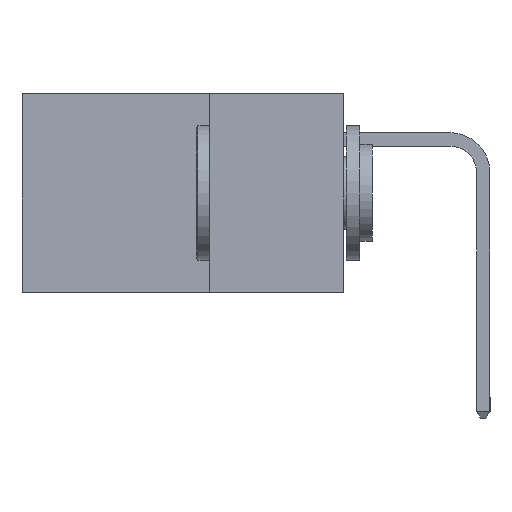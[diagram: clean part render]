
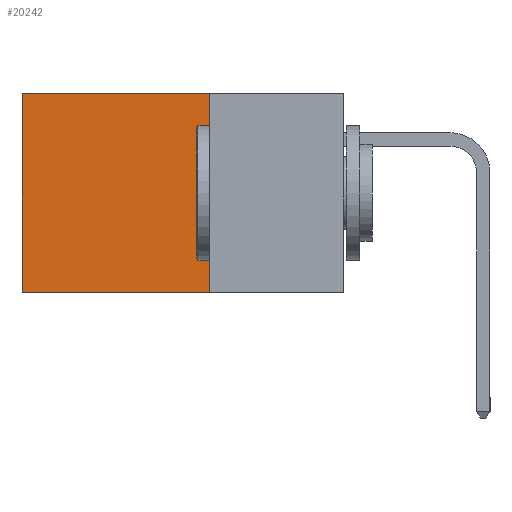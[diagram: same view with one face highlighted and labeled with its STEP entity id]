
A CAD part, left-side view. The second image highlights one B-rep face of the part: STEP entity #20242.
In plain terms, the highlighted planar face has unit normal (-1, 0, 0).
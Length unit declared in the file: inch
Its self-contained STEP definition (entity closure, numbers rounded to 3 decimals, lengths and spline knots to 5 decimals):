
#488 = CARTESIAN_POINT ( 'NONE',  ( 0.2615, 0.25, 0. ) ) ;
#850 = VERTEX_POINT ( 'NONE', #1772 ) ;
#869 = ORIENTED_EDGE ( 'NONE', *, *, #1968, .T. ) ;
#1075 = EDGE_LOOP ( 'NONE', ( #2644, #16100, #10027, #869 ) ) ;
#1772 = CARTESIAN_POINT ( 'NONE',  ( 0.2615, 0.25, 0. ) ) ;
#1968 = EDGE_CURVE ( 'NONE', #850, #8226, #18733, .T. ) ;
#2470 = AXIS2_PLACEMENT_3D ( 'NONE', #17367, #19118, #8888 ) ;
#2644 = ORIENTED_EDGE ( 'NONE', *, *, #14358, .T. ) ;
#3655 = CARTESIAN_POINT ( 'NONE',  ( 0.2615, 0.25, -0.37 ) ) ;
#5362 = PLANE ( 'NONE',  #2470 ) ;
#7744 = LINE ( 'NONE', #14779, #19752 ) ;
#8226 = VERTEX_POINT ( 'NONE', #15303 ) ;
#8234 = EDGE_CURVE ( 'NONE', #850, #11960, #7744, .T. ) ;
#8888 = DIRECTION ( 'NONE',  ( 0., 0., -1. ) ) ;
#9257 = VECTOR ( 'NONE', #21228, 39.37008 ) ;
#9648 = VECTOR ( 'NONE', #21677, 39.37008 ) ;
#10027 = ORIENTED_EDGE ( 'NONE', *, *, #8234, .F. ) ;
#11348 = DIRECTION ( 'NONE',  ( 0., 0., -1. ) ) ;
#11352 = CARTESIAN_POINT ( 'NONE',  ( 0.2615, 0.6, -0.37 ) ) ;
#11960 = VERTEX_POINT ( 'NONE', #3655 ) ;
#14358 = EDGE_CURVE ( 'NONE', #8226, #20676, #19273, .T. ) ;
#14633 = DIRECTION ( 'NONE',  ( 0., 0., -1. ) ) ;
#14745 = VECTOR ( 'NONE', #11348, 39.37008 ) ;
#14779 = CARTESIAN_POINT ( 'NONE',  ( 0.2615, 0.25, -0.37 ) ) ;
#15089 = EDGE_CURVE ( 'NONE', #11960, #20676, #18312, .T. ) ;
#15303 = CARTESIAN_POINT ( 'NONE',  ( 0.2615, 0.6, 0. ) ) ;
#16100 = ORIENTED_EDGE ( 'NONE', *, *, #15089, .F. ) ;
#17367 = CARTESIAN_POINT ( 'NONE',  ( 0.2615, 0.25, -0.37 ) ) ;
#18081 = FACE_OUTER_BOUND ( 'NONE', #1075, .T. ) ;
#18312 = LINE ( 'NONE', #21293, #9257 ) ;
#18561 = CARTESIAN_POINT ( 'NONE',  ( 0.2615, 0.6, -0.37 ) ) ;
#18733 = LINE ( 'NONE', #488, #9648 ) ;
#19118 = DIRECTION ( 'NONE',  ( 1., 0., 0. ) ) ;
#19273 = LINE ( 'NONE', #11352, #14745 ) ;
#19752 = VECTOR ( 'NONE', #14633, 39.37008 ) ;
#20242 = ADVANCED_FACE ( 'NONE', ( #18081 ), #5362, .F. ) ;
#20676 = VERTEX_POINT ( 'NONE', #18561 ) ;
#21228 = DIRECTION ( 'NONE',  ( 0., 1., 0. ) ) ;
#21293 = CARTESIAN_POINT ( 'NONE',  ( 0.2615, 0.25, -0.37 ) ) ;
#21677 = DIRECTION ( 'NONE',  ( 0., 1., 0. ) ) ;
